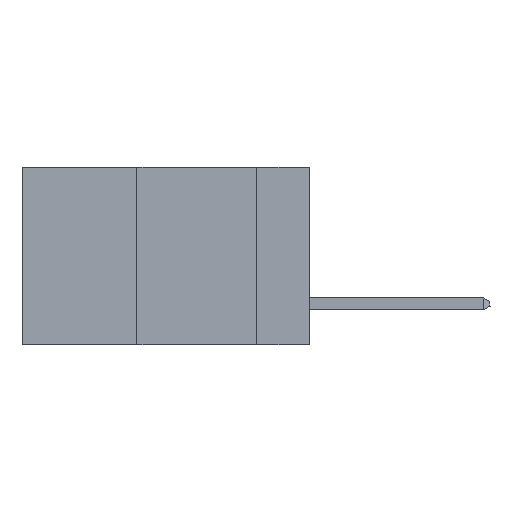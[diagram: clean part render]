
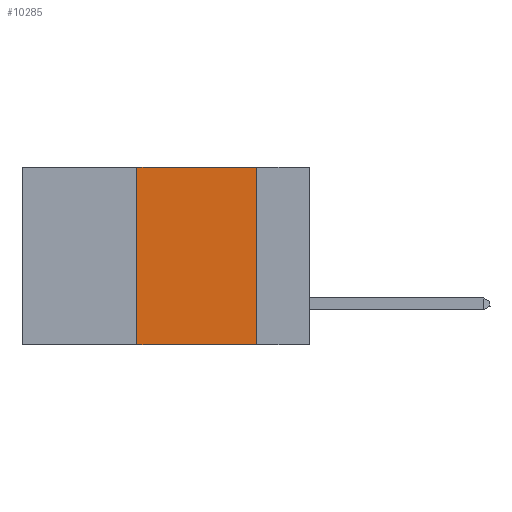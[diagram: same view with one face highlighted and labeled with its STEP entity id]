
A CAD part, left-side view. The second image highlights one B-rep face of the part: STEP entity #10285.
In plain terms, the highlighted planar face has unit normal (-1, 0, 0).
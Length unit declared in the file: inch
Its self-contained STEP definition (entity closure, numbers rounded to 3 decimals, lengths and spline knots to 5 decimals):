
#556 = LINE ( 'NONE', #2274, #3112 ) ;
#804 = VERTEX_POINT ( 'NONE', #13778 ) ;
#1207 = VERTEX_POINT ( 'NONE', #12982 ) ;
#1751 = VECTOR ( 'NONE', #7198, 39.37008 ) ;
#2274 = CARTESIAN_POINT ( 'NONE',  ( 0., 0.6, -0.37 ) ) ;
#3112 = VECTOR ( 'NONE', #16838, 39.37008 ) ;
#6442 = FACE_OUTER_BOUND ( 'NONE', #18482, .T. ) ;
#7041 = EDGE_CURVE ( 'NONE', #804, #1207, #11373, .T. ) ;
#7198 = DIRECTION ( 'NONE',  ( 0., 0., 1. ) ) ;
#8383 = EDGE_CURVE ( 'NONE', #16979, #1207, #556, .T. ) ;
#9013 = ORIENTED_EDGE ( 'NONE', *, *, #14301, .F. ) ;
#9270 = VERTEX_POINT ( 'NONE', #19151 ) ;
#9886 = PLANE ( 'NONE',  #19614 ) ;
#10285 = ADVANCED_FACE ( 'NONE', ( #6442 ), #9886, .F. ) ;
#11065 = DIRECTION ( 'NONE',  ( 0., 0., -1. ) ) ;
#11373 = LINE ( 'NONE', #19180, #20382 ) ;
#11412 = CARTESIAN_POINT ( 'NONE',  ( 0., 0.6, 0. ) ) ;
#11445 = DIRECTION ( 'NONE',  ( 0., 0., -1. ) ) ;
#12982 = CARTESIAN_POINT ( 'NONE',  ( 0., 0.11, -0.37 ) ) ;
#13116 = DIRECTION ( 'NONE',  ( 1., 0., 0. ) ) ;
#13778 = CARTESIAN_POINT ( 'NONE',  ( 0., 0.11, 0. ) ) ;
#14301 = EDGE_CURVE ( 'NONE', #9270, #804, #19320, .T. ) ;
#14351 = ORIENTED_EDGE ( 'NONE', *, *, #16617, .F. ) ;
#14437 = ORIENTED_EDGE ( 'NONE', *, *, #8383, .T. ) ;
#16373 = LINE ( 'NONE', #17015, #1751 ) ;
#16617 = EDGE_CURVE ( 'NONE', #16979, #9270, #16373, .T. ) ;
#16838 = DIRECTION ( 'NONE',  ( 0., -1., 0. ) ) ;
#16979 = VERTEX_POINT ( 'NONE', #19503 ) ;
#17015 = CARTESIAN_POINT ( 'NONE',  ( 0., 0.36, 0. ) ) ;
#17053 = ORIENTED_EDGE ( 'NONE', *, *, #7041, .F. ) ;
#18000 = CARTESIAN_POINT ( 'NONE',  ( 0., 0.6, 0. ) ) ;
#18280 = VECTOR ( 'NONE', #18313, 39.37008 ) ;
#18313 = DIRECTION ( 'NONE',  ( 0., -1., 0. ) ) ;
#18482 = EDGE_LOOP ( 'NONE', ( #17053, #9013, #14351, #14437 ) ) ;
#19151 = CARTESIAN_POINT ( 'NONE',  ( 0., 0.36, 0. ) ) ;
#19180 = CARTESIAN_POINT ( 'NONE',  ( 0., 0.11, 0. ) ) ;
#19320 = LINE ( 'NONE', #11412, #18280 ) ;
#19503 = CARTESIAN_POINT ( 'NONE',  ( 0., 0.36, -0.37 ) ) ;
#19614 = AXIS2_PLACEMENT_3D ( 'NONE', #18000, #13116, #11445 ) ;
#20382 = VECTOR ( 'NONE', #11065, 39.37008 ) ;
